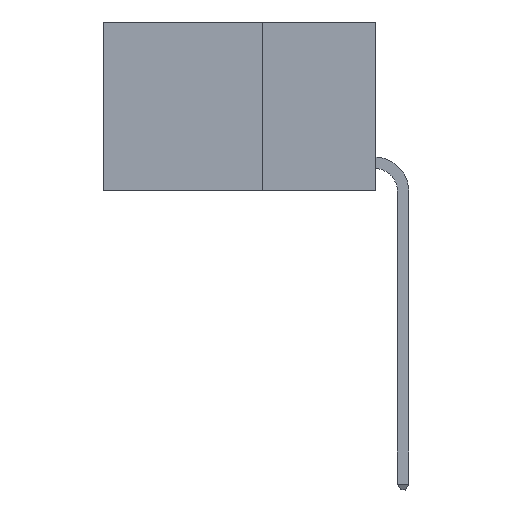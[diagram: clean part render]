
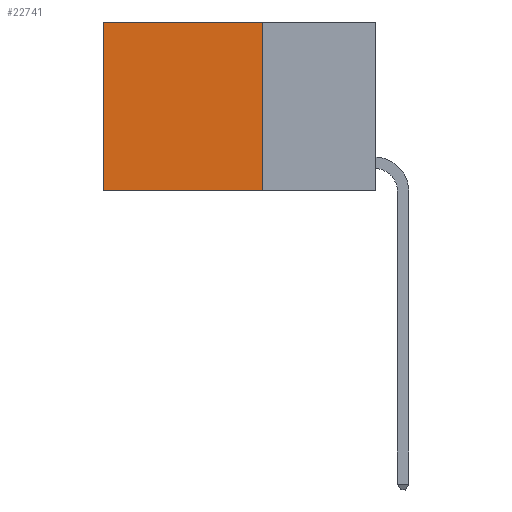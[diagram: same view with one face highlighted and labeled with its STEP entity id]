
A CAD part, left-side view. The second image highlights one B-rep face of the part: STEP entity #22741.
In plain terms, the highlighted planar face has unit normal (-1, 0, 0).
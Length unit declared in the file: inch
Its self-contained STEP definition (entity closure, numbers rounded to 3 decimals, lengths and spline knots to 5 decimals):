
#349 = VERTEX_POINT ( 'NONE', #14178 ) ;
#1811 = EDGE_CURVE ( 'NONE', #15267, #349, #15417, .T. ) ;
#1939 = LINE ( 'NONE', #10112, #24432 ) ;
#2204 = EDGE_LOOP ( 'NONE', ( #24351, #27030, #14328, #27414 ) ) ;
#2363 = DIRECTION ( 'NONE',  ( 0., 0., -1. ) ) ;
#3468 = AXIS2_PLACEMENT_3D ( 'NONE', #13451, #15649, #2363 ) ;
#3579 = CARTESIAN_POINT ( 'NONE',  ( 0.2625, 0.25, -0.37 ) ) ;
#6607 = LINE ( 'NONE', #3579, #22571 ) ;
#6718 = CARTESIAN_POINT ( 'NONE',  ( 0.2625, 0.6, 0. ) ) ;
#7969 = DIRECTION ( 'NONE',  ( 0., 1., 0. ) ) ;
#8974 = DIRECTION ( 'NONE',  ( 0., 0., -1. ) ) ;
#9884 = DIRECTION ( 'NONE',  ( 0., 0., -1. ) ) ;
#10112 = CARTESIAN_POINT ( 'NONE',  ( 0.2625, 0.25, 0. ) ) ;
#10305 = DIRECTION ( 'NONE',  ( 0., 1., 0. ) ) ;
#10396 = CARTESIAN_POINT ( 'NONE',  ( 0.2625, 0.25, 0. ) ) ;
#11852 = EDGE_CURVE ( 'NONE', #15150, #14943, #13743, .T. ) ;
#12530 = CARTESIAN_POINT ( 'NONE',  ( 0.2625, 0.25, 0. ) ) ;
#12694 = FACE_OUTER_BOUND ( 'NONE', #2204, .T. ) ;
#13451 = CARTESIAN_POINT ( 'NONE',  ( 0.2625, 0.25, 0. ) ) ;
#13743 = LINE ( 'NONE', #6718, #24393 ) ;
#14178 = CARTESIAN_POINT ( 'NONE',  ( 0.2625, 0.25, -0.37 ) ) ;
#14328 = ORIENTED_EDGE ( 'NONE', *, *, #1811, .F. ) ;
#14943 = VERTEX_POINT ( 'NONE', #24298 ) ;
#15150 = VERTEX_POINT ( 'NONE', #20726 ) ;
#15266 = EDGE_CURVE ( 'NONE', #349, #14943, #6607, .T. ) ;
#15267 = VERTEX_POINT ( 'NONE', #12530 ) ;
#15417 = LINE ( 'NONE', #10396, #19739 ) ;
#15649 = DIRECTION ( 'NONE',  ( 1., 0., 0. ) ) ;
#18368 = EDGE_CURVE ( 'NONE', #15267, #15150, #1939, .T. ) ;
#19739 = VECTOR ( 'NONE', #9884, 39.37008 ) ;
#20726 = CARTESIAN_POINT ( 'NONE',  ( 0.2625, 0.6, 0. ) ) ;
#22571 = VECTOR ( 'NONE', #10305, 39.37008 ) ;
#22741 = ADVANCED_FACE ( 'NONE', ( #12694 ), #26141, .F. ) ;
#24298 = CARTESIAN_POINT ( 'NONE',  ( 0.2625, 0.6, -0.37 ) ) ;
#24351 = ORIENTED_EDGE ( 'NONE', *, *, #11852, .T. ) ;
#24393 = VECTOR ( 'NONE', #8974, 39.37008 ) ;
#24432 = VECTOR ( 'NONE', #7969, 39.37008 ) ;
#26141 = PLANE ( 'NONE',  #3468 ) ;
#27030 = ORIENTED_EDGE ( 'NONE', *, *, #15266, .F. ) ;
#27414 = ORIENTED_EDGE ( 'NONE', *, *, #18368, .T. ) ;
